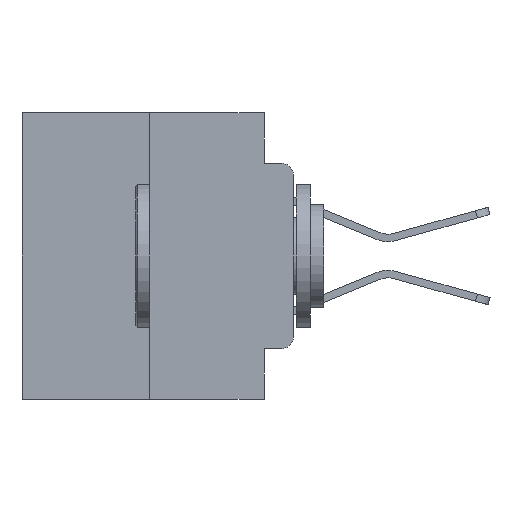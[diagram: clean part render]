
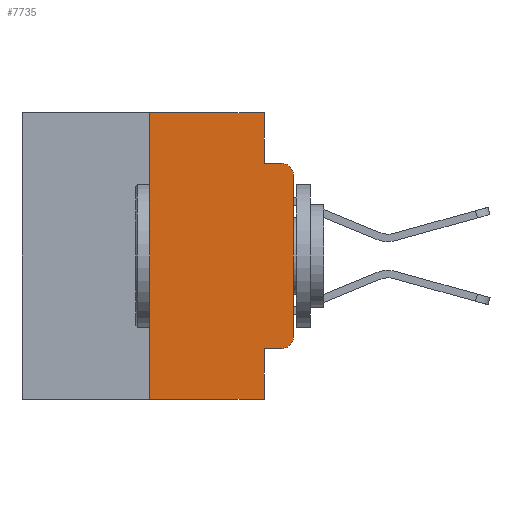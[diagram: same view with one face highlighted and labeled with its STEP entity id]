
A CAD part, left-side view. The second image highlights one B-rep face of the part: STEP entity #7735.
In plain terms, the highlighted planar face has unit normal (-1, 0, 0).
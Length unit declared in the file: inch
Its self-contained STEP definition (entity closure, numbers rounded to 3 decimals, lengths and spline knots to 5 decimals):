
#147 = ORIENTED_EDGE ( 'NONE', *, *, #20108, .T. ) ;
#305 = ORIENTED_EDGE ( 'NONE', *, *, #21243, .F. ) ;
#306 = PLANE ( 'NONE',  #8693 ) ;
#360 = ORIENTED_EDGE ( 'NONE', *, *, #8350, .F. ) ;
#397 = DIRECTION ( 'NONE',  ( 0., 0., 1. ) ) ;
#1813 = VECTOR ( 'NONE', #18729, 39.37008 ) ;
#2146 = LINE ( 'NONE', #25720, #1813 ) ;
#2494 = VERTEX_POINT ( 'NONE', #2822 ) ;
#2570 = CARTESIAN_POINT ( 'NONE',  ( 0., 0.473, 0. ) ) ;
#2822 = CARTESIAN_POINT ( 'NONE',  ( 0., 0.02, -0.4115 ) ) ;
#2845 = VECTOR ( 'NONE', #397, 39.37008 ) ;
#2976 = FACE_OUTER_BOUND ( 'NONE', #13055, .T. ) ;
#3286 = ORIENTED_EDGE ( 'NONE', *, *, #21955, .T. ) ;
#4020 = EDGE_CURVE ( 'NONE', #21193, #15941, #2146, .T. ) ;
#4627 = LINE ( 'NONE', #28188, #13969 ) ;
#5189 = ORIENTED_EDGE ( 'NONE', *, *, #21455, .F. ) ;
#6360 = LINE ( 'NONE', #23200, #12940 ) ;
#6724 = DIRECTION ( 'NONE',  ( 0., 0., -1. ) ) ;
#7184 = DIRECTION ( 'NONE',  ( -1., 0., 0. ) ) ;
#7216 = VERTEX_POINT ( 'NONE', #22323 ) ;
#7735 = ADVANCED_FACE ( 'NONE', ( #2976 ), #306, .F. ) ;
#8274 = VECTOR ( 'NONE', #10373, 39.37008 ) ;
#8350 = EDGE_CURVE ( 'NONE', #14593, #23202, #24690, .T. ) ;
#8457 = DIRECTION ( 'NONE',  ( 0., 0., 1. ) ) ;
#8529 = CARTESIAN_POINT ( 'NONE',  ( 0., 0., -0.3915 ) ) ;
#8548 = CIRCLE ( 'NONE', #19483, 0.02 ) ;
#8693 = AXIS2_PLACEMENT_3D ( 'NONE', #9151, #13488, #6724 ) ;
#9151 = CARTESIAN_POINT ( 'NONE',  ( 0., 0.473, 0. ) ) ;
#9222 = DIRECTION ( 'NONE',  ( 0., 0., -1. ) ) ;
#9258 = DIRECTION ( 'NONE',  ( 0., -1., 0. ) ) ;
#9307 = DIRECTION ( 'NONE',  ( 0., -1., 0. ) ) ;
#10373 = DIRECTION ( 'NONE',  ( 0., -1., 0. ) ) ;
#10575 = VECTOR ( 'NONE', #21053, 39.37008 ) ;
#11367 = CARTESIAN_POINT ( 'NONE',  ( 0., 0., 0. ) ) ;
#11425 = CIRCLE ( 'NONE', #13403, 0.02 ) ;
#11845 = CARTESIAN_POINT ( 'NONE',  ( 0., 0.25, 0. ) ) ;
#12115 = CARTESIAN_POINT ( 'NONE',  ( 0., 0.25, -0.5 ) ) ;
#12311 = LINE ( 'NONE', #22301, #20956 ) ;
#12940 = VECTOR ( 'NONE', #9307, 39.37008 ) ;
#13055 = EDGE_LOOP ( 'NONE', ( #3286, #18002, #5189, #360, #16024, #305, #147, #27051, #24869, #14821 ) ) ;
#13403 = AXIS2_PLACEMENT_3D ( 'NONE', #21589, #26172, #19570 ) ;
#13488 = DIRECTION ( 'NONE',  ( 1., 0., 0. ) ) ;
#13969 = VECTOR ( 'NONE', #8457, 39.37008 ) ;
#14336 = CARTESIAN_POINT ( 'NONE',  ( 0., 0.051, -0.5 ) ) ;
#14421 = EDGE_CURVE ( 'NONE', #17763, #14593, #20264, .T. ) ;
#14593 = VERTEX_POINT ( 'NONE', #21133 ) ;
#14611 = LINE ( 'NONE', #11367, #2845 ) ;
#14821 = ORIENTED_EDGE ( 'NONE', *, *, #28080, .T. ) ;
#15016 = CARTESIAN_POINT ( 'NONE',  ( 0., 0.051, -0.4115 ) ) ;
#15757 = DIRECTION ( 'NONE',  ( 0., -1., 0. ) ) ;
#15941 = VERTEX_POINT ( 'NONE', #14336 ) ;
#15974 = CARTESIAN_POINT ( 'NONE',  ( 0., 0.02, -0.3915 ) ) ;
#16024 = ORIENTED_EDGE ( 'NONE', *, *, #14421, .F. ) ;
#17763 = VERTEX_POINT ( 'NONE', #11845 ) ;
#18002 = ORIENTED_EDGE ( 'NONE', *, *, #23361, .T. ) ;
#18729 = DIRECTION ( 'NONE',  ( 0., 0., -1. ) ) ;
#19103 = CARTESIAN_POINT ( 'NONE',  ( 0., 0.051, 0. ) ) ;
#19483 = AXIS2_PLACEMENT_3D ( 'NONE', #15974, #7184, #9222 ) ;
#19570 = DIRECTION ( 'NONE',  ( 0., 0., -1. ) ) ;
#19842 = VERTEX_POINT ( 'NONE', #12115 ) ;
#20108 = EDGE_CURVE ( 'NONE', #19842, #15941, #12311, .T. ) ;
#20264 = LINE ( 'NONE', #2570, #26765 ) ;
#20613 = CARTESIAN_POINT ( 'NONE',  ( 0., 0.02, -0.0885 ) ) ;
#20956 = VECTOR ( 'NONE', #15757, 39.37008 ) ;
#21053 = DIRECTION ( 'NONE',  ( 0., 0., -1. ) ) ;
#21082 = LINE ( 'NONE', #21278, #8274 ) ;
#21133 = CARTESIAN_POINT ( 'NONE',  ( 0., 0.051, 0. ) ) ;
#21193 = VERTEX_POINT ( 'NONE', #15016 ) ;
#21243 = EDGE_CURVE ( 'NONE', #19842, #17763, #4627, .T. ) ;
#21278 = CARTESIAN_POINT ( 'NONE',  ( 0., 0.051, -0.4115 ) ) ;
#21455 = EDGE_CURVE ( 'NONE', #23202, #28185, #6360, .T. ) ;
#21589 = CARTESIAN_POINT ( 'NONE',  ( 0., 0.02, -0.1085 ) ) ;
#21955 = EDGE_CURVE ( 'NONE', #24052, #7216, #14611, .T. ) ;
#22301 = CARTESIAN_POINT ( 'NONE',  ( 0., 0.473, -0.5 ) ) ;
#22323 = CARTESIAN_POINT ( 'NONE',  ( 0., 0., -0.1085 ) ) ;
#22650 = CARTESIAN_POINT ( 'NONE',  ( 0., 0.051, -0.0885 ) ) ;
#23200 = CARTESIAN_POINT ( 'NONE',  ( 0., 0.051, -0.0885 ) ) ;
#23202 = VERTEX_POINT ( 'NONE', #22650 ) ;
#23361 = EDGE_CURVE ( 'NONE', #7216, #28185, #11425, .T. ) ;
#23972 = EDGE_CURVE ( 'NONE', #21193, #2494, #21082, .T. ) ;
#24052 = VERTEX_POINT ( 'NONE', #8529 ) ;
#24690 = LINE ( 'NONE', #19103, #10575 ) ;
#24869 = ORIENTED_EDGE ( 'NONE', *, *, #23972, .T. ) ;
#25720 = CARTESIAN_POINT ( 'NONE',  ( 0., 0.051, 0. ) ) ;
#26172 = DIRECTION ( 'NONE',  ( -1., 0., 0. ) ) ;
#26765 = VECTOR ( 'NONE', #9258, 39.37008 ) ;
#27051 = ORIENTED_EDGE ( 'NONE', *, *, #4020, .F. ) ;
#28080 = EDGE_CURVE ( 'NONE', #2494, #24052, #8548, .T. ) ;
#28185 = VERTEX_POINT ( 'NONE', #20613 ) ;
#28188 = CARTESIAN_POINT ( 'NONE',  ( 0., 0.25, 0. ) ) ;
